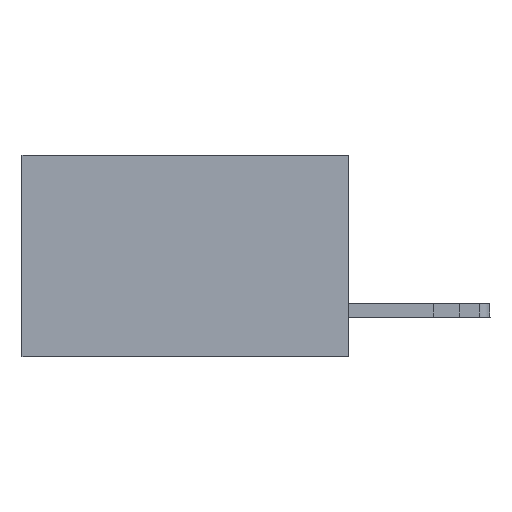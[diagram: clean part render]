
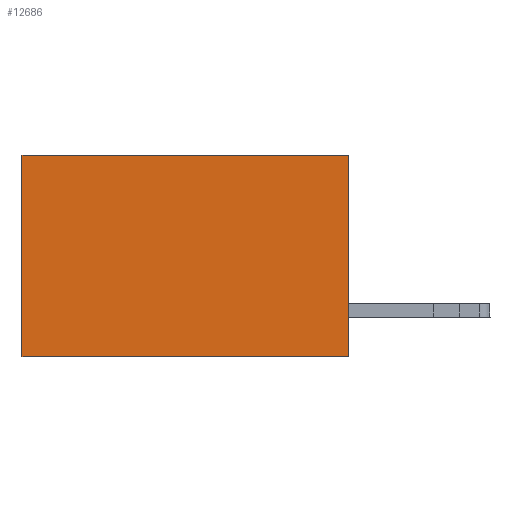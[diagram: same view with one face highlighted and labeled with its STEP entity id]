
A CAD part, left-side view. The second image highlights one B-rep face of the part: STEP entity #12686.
In plain terms, the highlighted planar face has unit normal (-1, 0, 0).
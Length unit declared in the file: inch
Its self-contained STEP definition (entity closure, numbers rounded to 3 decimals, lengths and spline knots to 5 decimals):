
#637 = VERTEX_POINT ( 'NONE', #4147 ) ;
#1723 = VERTEX_POINT ( 'NONE', #21626 ) ;
#3615 = CARTESIAN_POINT ( 'NONE',  ( 0.298, 0., 0. ) ) ;
#3635 = EDGE_CURVE ( 'NONE', #5039, #1723, #10575, .T. ) ;
#4027 = EDGE_CURVE ( 'NONE', #1723, #5135, #20792, .T. ) ;
#4147 = CARTESIAN_POINT ( 'NONE',  ( 0.298, 0., -0.37 ) ) ;
#4921 = DIRECTION ( 'NONE',  ( 0., 1., 0. ) ) ;
#5039 = VERTEX_POINT ( 'NONE', #21006 ) ;
#5135 = VERTEX_POINT ( 'NONE', #23965 ) ;
#5377 = CARTESIAN_POINT ( 'NONE',  ( 0.298, 0., 0. ) ) ;
#5969 = DIRECTION ( 'NONE',  ( 0., 0., -1. ) ) ;
#6272 = CARTESIAN_POINT ( 'NONE',  ( 0.298, 0., 0. ) ) ;
#6934 = VECTOR ( 'NONE', #15963, 39.37008 ) ;
#7345 = FACE_OUTER_BOUND ( 'NONE', #23073, .T. ) ;
#8066 = ORIENTED_EDGE ( 'NONE', *, *, #4027, .T. ) ;
#9301 = AXIS2_PLACEMENT_3D ( 'NONE', #3615, #26717, #5969 ) ;
#10575 = LINE ( 'NONE', #5377, #6934 ) ;
#10816 = ORIENTED_EDGE ( 'NONE', *, *, #3635, .T. ) ;
#12538 = EDGE_CURVE ( 'NONE', #5039, #637, #25778, .T. ) ;
#12686 = ADVANCED_FACE ( 'NONE', ( #7345 ), #24599, .F. ) ;
#14354 = VECTOR ( 'NONE', #4921, 39.37008 ) ;
#15190 = VECTOR ( 'NONE', #25071, 39.37008 ) ;
#15963 = DIRECTION ( 'NONE',  ( 0., 1., 0. ) ) ;
#17521 = DIRECTION ( 'NONE',  ( 0., 0., -1. ) ) ;
#19629 = CARTESIAN_POINT ( 'NONE',  ( 0.298, 0., -0.37 ) ) ;
#20639 = ORIENTED_EDGE ( 'NONE', *, *, #12538, .F. ) ;
#20792 = LINE ( 'NONE', #26821, #15190 ) ;
#21006 = CARTESIAN_POINT ( 'NONE',  ( 0.298, 0., 0. ) ) ;
#21209 = ORIENTED_EDGE ( 'NONE', *, *, #27192, .F. ) ;
#21279 = LINE ( 'NONE', #19629, #14354 ) ;
#21626 = CARTESIAN_POINT ( 'NONE',  ( 0.298, 0.6, 0. ) ) ;
#22533 = VECTOR ( 'NONE', #17521, 39.37008 ) ;
#23073 = EDGE_LOOP ( 'NONE', ( #8066, #21209, #20639, #10816 ) ) ;
#23965 = CARTESIAN_POINT ( 'NONE',  ( 0.298, 0.6, -0.37 ) ) ;
#24599 = PLANE ( 'NONE',  #9301 ) ;
#25071 = DIRECTION ( 'NONE',  ( 0., 0., -1. ) ) ;
#25778 = LINE ( 'NONE', #6272, #22533 ) ;
#26717 = DIRECTION ( 'NONE',  ( 1., 0., 0. ) ) ;
#26821 = CARTESIAN_POINT ( 'NONE',  ( 0.298, 0.6, 0. ) ) ;
#27192 = EDGE_CURVE ( 'NONE', #637, #5135, #21279, .T. ) ;
